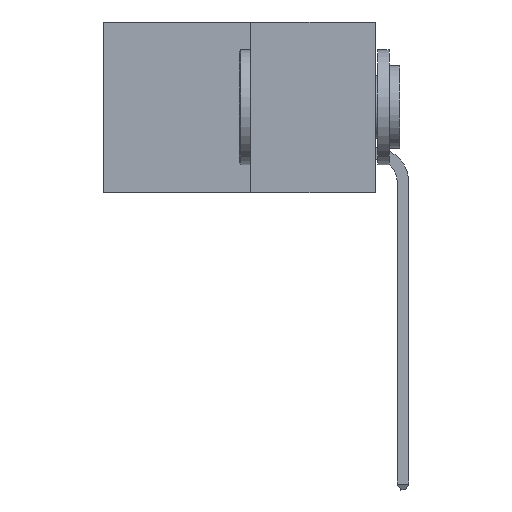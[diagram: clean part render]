
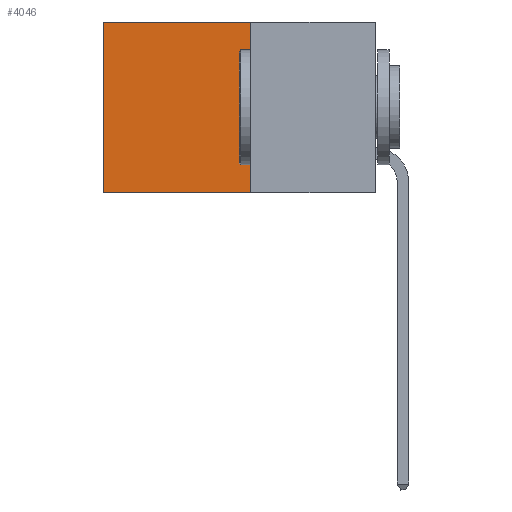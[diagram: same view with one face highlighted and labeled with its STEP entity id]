
A CAD part, left-side view. The second image highlights one B-rep face of the part: STEP entity #4046.
In plain terms, the highlighted planar face has unit normal (-1, 0, 0).
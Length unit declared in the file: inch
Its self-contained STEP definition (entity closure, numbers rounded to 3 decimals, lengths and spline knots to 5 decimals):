
#107 = VERTEX_POINT ( 'NONE', #3853 ) ;
#231 = DIRECTION ( 'NONE',  ( 0., 0., -1. ) ) ;
#368 = DIRECTION ( 'NONE',  ( 1., 0., 0. ) ) ;
#447 = DIRECTION ( 'NONE',  ( 0., 1., 0. ) ) ;
#496 = AXIS2_PLACEMENT_3D ( 'NONE', #503, #368, #231 ) ;
#503 = CARTESIAN_POINT ( 'NONE',  ( 0.277, 0.27, -0.37 ) ) ;
#514 = PLANE ( 'NONE',  #496 ) ;
#789 = CARTESIAN_POINT ( 'NONE',  ( 0.277, 0.27, -0.37 ) ) ;
#1846 = EDGE_CURVE ( 'NONE', #9699, #10735, #2553, .T. ) ;
#2271 = VECTOR ( 'NONE', #447, 39.37008 ) ;
#2553 = LINE ( 'NONE', #7185, #2271 ) ;
#3138 = EDGE_CURVE ( 'NONE', #8409, #107, #10653, .T. ) ;
#3403 = ORIENTED_EDGE ( 'NONE', *, *, #10434, .T. ) ;
#3853 = CARTESIAN_POINT ( 'NONE',  ( 0.277, 0.59, -0.37 ) ) ;
#3943 = ORIENTED_EDGE ( 'NONE', *, *, #1846, .T. ) ;
#4045 = VECTOR ( 'NONE', #11194, 39.37008 ) ;
#4046 = ADVANCED_FACE ( 'NONE', ( #10876 ), #514, .F. ) ;
#4210 = CARTESIAN_POINT ( 'NONE',  ( 0.277, 0.59, -0.37 ) ) ;
#4993 = VECTOR ( 'NONE', #9219, 39.37008 ) ;
#5193 = EDGE_LOOP ( 'NONE', ( #3403, #7943, #10327, #3943 ) ) ;
#5258 = LINE ( 'NONE', #4210, #4993 ) ;
#5263 = LINE ( 'NONE', #10733, #6999 ) ;
#5545 = CARTESIAN_POINT ( 'NONE',  ( 0.277, 0.27, 0. ) ) ;
#5942 = CARTESIAN_POINT ( 'NONE',  ( 0.277, 0.27, -0.37 ) ) ;
#6999 = VECTOR ( 'NONE', #7518, 39.37008 ) ;
#7185 = CARTESIAN_POINT ( 'NONE',  ( 0.277, 0.27, 0. ) ) ;
#7518 = DIRECTION ( 'NONE',  ( 0., 0., -1. ) ) ;
#7943 = ORIENTED_EDGE ( 'NONE', *, *, #3138, .F. ) ;
#8409 = VERTEX_POINT ( 'NONE', #789 ) ;
#8854 = CARTESIAN_POINT ( 'NONE',  ( 0.277, 0.59, 0. ) ) ;
#9219 = DIRECTION ( 'NONE',  ( 0., 0., -1. ) ) ;
#9364 = EDGE_CURVE ( 'NONE', #9699, #8409, #5263, .T. ) ;
#9699 = VERTEX_POINT ( 'NONE', #5545 ) ;
#10327 = ORIENTED_EDGE ( 'NONE', *, *, #9364, .F. ) ;
#10434 = EDGE_CURVE ( 'NONE', #10735, #107, #5258, .T. ) ;
#10653 = LINE ( 'NONE', #5942, #4045 ) ;
#10733 = CARTESIAN_POINT ( 'NONE',  ( 0.277, 0.27, -0.37 ) ) ;
#10735 = VERTEX_POINT ( 'NONE', #8854 ) ;
#10876 = FACE_OUTER_BOUND ( 'NONE', #5193, .T. ) ;
#11194 = DIRECTION ( 'NONE',  ( 0., 1., 0. ) ) ;
